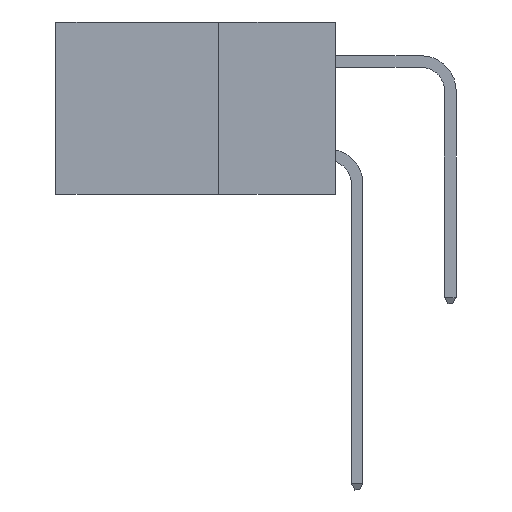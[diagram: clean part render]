
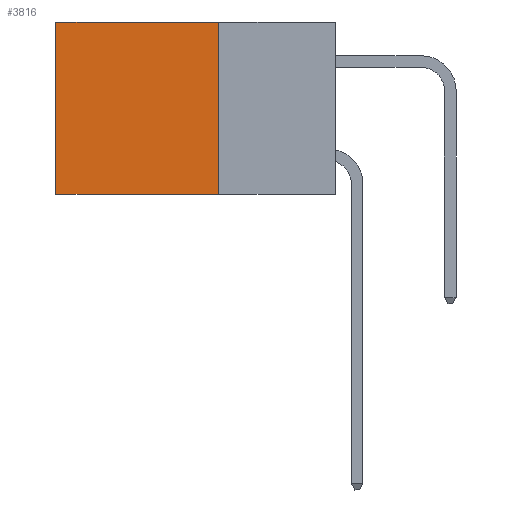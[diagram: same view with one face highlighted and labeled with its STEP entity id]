
A CAD part, left-side view. The second image highlights one B-rep face of the part: STEP entity #3816.
In plain terms, the highlighted planar face has unit normal (-1, 0, 0).
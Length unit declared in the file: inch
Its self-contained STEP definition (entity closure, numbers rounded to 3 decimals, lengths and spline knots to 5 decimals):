
#135 = ORIENTED_EDGE ( 'NONE', *, *, #29702, .T. ) ;
#1566 = VECTOR ( 'NONE', #3224, 39.37008 ) ;
#3224 = DIRECTION ( 'NONE',  ( 0., 0., -1. ) ) ;
#3816 = ADVANCED_FACE ( 'NONE', ( #25692 ), #8119, .F. ) ;
#4999 = DIRECTION ( 'NONE',  ( 0., 1., 0. ) ) ;
#5081 = VERTEX_POINT ( 'NONE', #30935 ) ;
#5712 = LINE ( 'NONE', #20464, #25372 ) ;
#8119 = PLANE ( 'NONE',  #31195 ) ;
#8869 = VECTOR ( 'NONE', #4999, 39.37008 ) ;
#10144 = VERTEX_POINT ( 'NONE', #24164 ) ;
#10253 = DIRECTION ( 'NONE',  ( 0., 1., 0. ) ) ;
#10826 = CARTESIAN_POINT ( 'NONE',  ( 0.2875, 0.25, 0. ) ) ;
#12514 = VECTOR ( 'NONE', #23322, 39.37008 ) ;
#12718 = CARTESIAN_POINT ( 'NONE',  ( 0.2875, 0.25, -0.37 ) ) ;
#14806 = EDGE_CURVE ( 'NONE', #10144, #22592, #5712, .T. ) ;
#16116 = ORIENTED_EDGE ( 'NONE', *, *, #29629, .F. ) ;
#17296 = DIRECTION ( 'NONE',  ( 0., 0., -1. ) ) ;
#18650 = CARTESIAN_POINT ( 'NONE',  ( 0.2875, 0.6, 0. ) ) ;
#18732 = EDGE_CURVE ( 'NONE', #10144, #5081, #26092, .T. ) ;
#19029 = EDGE_LOOP ( 'NONE', ( #135, #16116, #22491, #32191 ) ) ;
#20464 = CARTESIAN_POINT ( 'NONE',  ( 0.2875, 0.25, 0. ) ) ;
#22491 = ORIENTED_EDGE ( 'NONE', *, *, #18732, .F. ) ;
#22592 = VERTEX_POINT ( 'NONE', #18650 ) ;
#23322 = DIRECTION ( 'NONE',  ( 0., 0., -1. ) ) ;
#24164 = CARTESIAN_POINT ( 'NONE',  ( 0.2875, 0.25, 0. ) ) ;
#25294 = CARTESIAN_POINT ( 'NONE',  ( 0.2875, 0.25, 0. ) ) ;
#25372 = VECTOR ( 'NONE', #10253, 39.37008 ) ;
#25692 = FACE_OUTER_BOUND ( 'NONE', #19029, .T. ) ;
#25914 = VERTEX_POINT ( 'NONE', #32544 ) ;
#26092 = LINE ( 'NONE', #10826, #1566 ) ;
#26905 = LINE ( 'NONE', #30892, #12514 ) ;
#27446 = DIRECTION ( 'NONE',  ( 1., 0., 0. ) ) ;
#27739 = LINE ( 'NONE', #12718, #8869 ) ;
#29629 = EDGE_CURVE ( 'NONE', #5081, #25914, #27739, .T. ) ;
#29702 = EDGE_CURVE ( 'NONE', #22592, #25914, #26905, .T. ) ;
#30892 = CARTESIAN_POINT ( 'NONE',  ( 0.2875, 0.6, 0. ) ) ;
#30935 = CARTESIAN_POINT ( 'NONE',  ( 0.2875, 0.25, -0.37 ) ) ;
#31195 = AXIS2_PLACEMENT_3D ( 'NONE', #25294, #27446, #17296 ) ;
#32191 = ORIENTED_EDGE ( 'NONE', *, *, #14806, .T. ) ;
#32544 = CARTESIAN_POINT ( 'NONE',  ( 0.2875, 0.6, -0.37 ) ) ;
